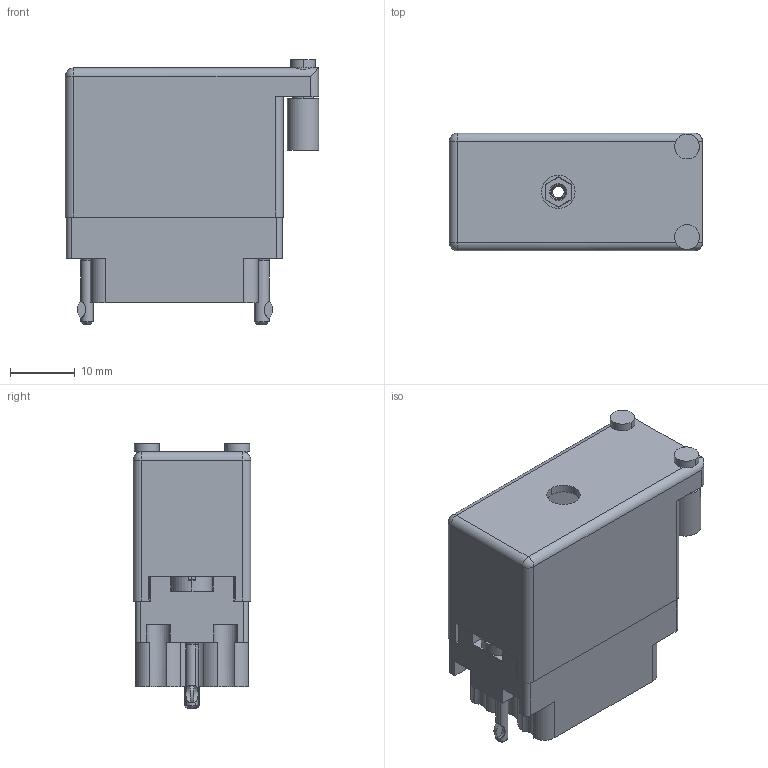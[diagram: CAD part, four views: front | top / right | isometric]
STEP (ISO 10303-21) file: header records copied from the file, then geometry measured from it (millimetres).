
FILE_DESCRIPTION (( 'STEP AP203' ), '1' );
FILE_NAME ('519-014-501-352.STEP', '2020-09-09T15:30:36', ( '' ), ( '' ), 'SwSTEP 2.0', 'SolidWorks 2020', '' );
FILE_SCHEMA (( 'CONFIG_CONTROL_DESIGN' ));
Length unit declared in the file: inch
Products named in the file (8): 516-222-020-102_014; 516-222-020-102_015; 516-230-001_Metal - 020 Side Entry; 519 Plug Insulator_014; 516-252-021-102_014; 519-014-501-352; 516-292-001_501 Contact; 516-252-025-100_516-252-025-100
Assembly tree (21 placements, depth 2):
  519-014-501-352
    519 Plug Insulator_014
    516-292-001_501 Contact  x14
    516-252-025-100_516-252-025-100
    516-252-021-102_014  x2
    516-222-020-102_014
    516-222-020-102_015
    516-230-001_Metal - 020 Side Entry
Bounding box: 39.12 x 18.16 x 40.84 mm (x, y, z)
Volume: 9795.6 mm3; surface area: 15489.2 mm2
Topology: 21 solids, 21 shells, 1814 faces, 5172 edges, 3412 vertices
Faces by surface type: plane 991, cylinder 645, bspline 123, cone 49, torus 4, sphere 2
Entity records: 35628 total; most frequent: CARTESIAN_POINT 12582, ORIENTED_EDGE 4752, DIRECTION 4416, EDGE_CURVE 2376, VERTEX_POINT 1558, AXIS2_PLACEMENT_3D 1480, VECTOR 1456, LINE 1456
